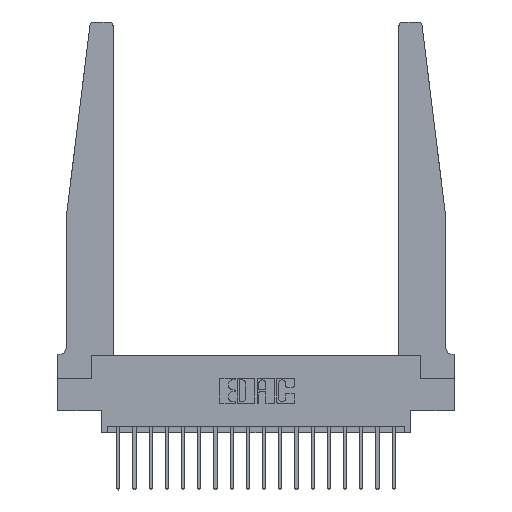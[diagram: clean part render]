
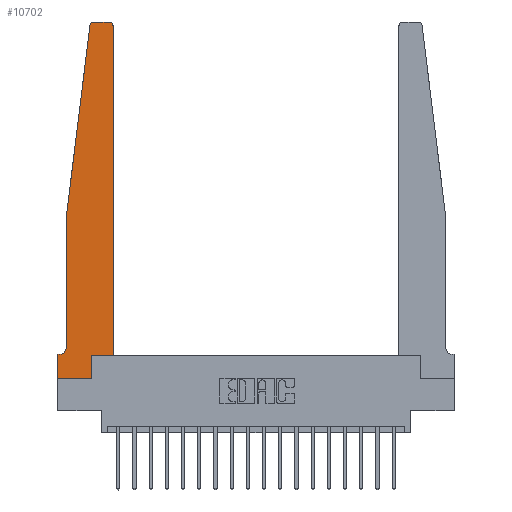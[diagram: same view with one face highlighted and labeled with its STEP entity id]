
A CAD part, top view. The second image highlights one B-rep face of the part: STEP entity #10702.
In plain terms, the highlighted planar face has unit normal (0, 0, 1).
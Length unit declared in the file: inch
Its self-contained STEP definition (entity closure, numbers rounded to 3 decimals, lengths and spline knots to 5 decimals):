
#874 = DIRECTION ( 'NONE',  ( -1., 0., 0. ) ) ;
#883 = VERTEX_POINT ( 'NONE', #2435 ) ;
#972 = CARTESIAN_POINT ( 'NONE',  ( 0., 0., 0.37 ) ) ;
#1206 = CARTESIAN_POINT ( 'NONE',  ( 0.065, 1.25, 0.37 ) ) ;
#1509 = CARTESIAN_POINT ( 'NONE',  ( 0.425, 0.18, 0.37 ) ) ;
#1638 = CARTESIAN_POINT ( 'NONE',  ( 0., 0.1875, 0.37 ) ) ;
#1744 = FACE_OUTER_BOUND ( 'NONE', #10239, .T. ) ;
#2054 = VECTOR ( 'NONE', #4395, 39.37008 ) ;
#2435 = CARTESIAN_POINT ( 'NONE',  ( 0.24675, 2.72367, 0.37 ) ) ;
#2833 = ORIENTED_EDGE ( 'NONE', *, *, #9319, .T. ) ;
#2853 = CARTESIAN_POINT ( 'NONE',  ( 0.425, 0.18, 0.37 ) ) ;
#2883 = LINE ( 'NONE', #19296, #9611 ) ;
#3149 = VECTOR ( 'NONE', #13732, 39.37008 ) ;
#3194 = DIRECTION ( 'NONE',  ( 1., 0., 0. ) ) ;
#3276 = CARTESIAN_POINT ( 'NONE',  ( 0.27653, 2.75, 0.37 ) ) ;
#3816 = ORIENTED_EDGE ( 'NONE', *, *, #16054, .T. ) ;
#4309 = VECTOR ( 'NONE', #18836, 39.37008 ) ;
#4395 = DIRECTION ( 'NONE',  ( 0., -1., 0. ) ) ;
#4402 = EDGE_CURVE ( 'NONE', #883, #15186, #13117, .T. ) ;
#4779 = AXIS2_PLACEMENT_3D ( 'NONE', #1638, #12386, #3194 ) ;
#5015 = ORIENTED_EDGE ( 'NONE', *, *, #6619, .T. ) ;
#5163 = CARTESIAN_POINT ( 'NONE',  ( 0.395, 2.72, 0.37 ) ) ;
#5362 = CARTESIAN_POINT ( 'NONE',  ( 0.27653, 2.72, 0.37 ) ) ;
#5660 = LINE ( 'NONE', #1206, #17437 ) ;
#5777 = CARTESIAN_POINT ( 'NONE',  ( 0.2605, 0.18, 0.37 ) ) ;
#5812 = CARTESIAN_POINT ( 'NONE',  ( 0.015, 0.2375, 0.37 ) ) ;
#5815 = EDGE_CURVE ( 'NONE', #15186, #13095, #5660, .T. ) ;
#5860 = CARTESIAN_POINT ( 'NONE',  ( 0., 0.1875, 0.37 ) ) ;
#6058 = CARTESIAN_POINT ( 'NONE',  ( 0.2605, 0., 0.37 ) ) ;
#6157 = VERTEX_POINT ( 'NONE', #19518 ) ;
#6160 = LINE ( 'NONE', #12027, #2054 ) ;
#6489 = CARTESIAN_POINT ( 'NONE',  ( 0.015, 0.1875, 0.37 ) ) ;
#6619 = EDGE_CURVE ( 'NONE', #15653, #883, #12093, .T. ) ;
#6700 = DIRECTION ( 'NONE',  ( 1., 0., 0. ) ) ;
#6887 = DIRECTION ( 'NONE',  ( 1., 0., 0. ) ) ;
#7202 = VECTOR ( 'NONE', #16511, 39.37008 ) ;
#7350 = DIRECTION ( 'NONE',  ( -1., 0., 0. ) ) ;
#7515 = DIRECTION ( 'NONE',  ( 1., 0., 0. ) ) ;
#7751 = LINE ( 'NONE', #12172, #3149 ) ;
#7836 = EDGE_CURVE ( 'NONE', #10323, #9070, #15899, .T. ) ;
#7864 = EDGE_CURVE ( 'NONE', #6157, #15653, #7751, .T. ) ;
#7906 = LINE ( 'NONE', #17312, #4309 ) ;
#8312 = EDGE_CURVE ( 'NONE', #13095, #19140, #11800, .T. ) ;
#8371 = EDGE_CURVE ( 'NONE', #8927, #10507, #6160, .T. ) ;
#8393 = ORIENTED_EDGE ( 'NONE', *, *, #16707, .T. ) ;
#8426 = VERTEX_POINT ( 'NONE', #6058 ) ;
#8843 = LINE ( 'NONE', #18296, #17024 ) ;
#8864 = ORIENTED_EDGE ( 'NONE', *, *, #15495, .T. ) ;
#8927 = VERTEX_POINT ( 'NONE', #5860 ) ;
#9070 = VERTEX_POINT ( 'NONE', #1509 ) ;
#9095 = DIRECTION ( 'NONE',  ( 1., 0., 0. ) ) ;
#9319 = EDGE_CURVE ( 'NONE', #16487, #6157, #14566, .T. ) ;
#9476 = CARTESIAN_POINT ( 'NONE',  ( 0.065, 0.2375, 0.37 ) ) ;
#9611 = VECTOR ( 'NONE', #874, 39.37008 ) ;
#10239 = EDGE_LOOP ( 'NONE', ( #13647, #5015, #16781, #12194, #19846, #8864, #12434, #8393, #3816, #19637, #15107, #2833 ) ) ;
#10323 = VERTEX_POINT ( 'NONE', #11480 ) ;
#10396 = DIRECTION ( 'NONE',  ( -0.122, -0.992, 0. ) ) ;
#10507 = VERTEX_POINT ( 'NONE', #972 ) ;
#10702 = ADVANCED_FACE ( 'NONE', ( #1744 ), #12323, .T. ) ;
#10782 = LINE ( 'NONE', #5777, #7202 ) ;
#11480 = CARTESIAN_POINT ( 'NONE',  ( 0.2605, 0.18, 0.37 ) ) ;
#11800 = CIRCLE ( 'NONE', #16057, 0.05 ) ;
#11821 = VECTOR ( 'NONE', #7515, 39.37008 ) ;
#12027 = CARTESIAN_POINT ( 'NONE',  ( 0., 0., 0.37 ) ) ;
#12093 = CIRCLE ( 'NONE', #17711, 0.03 ) ;
#12142 = VECTOR ( 'NONE', #10396, 39.37008 ) ;
#12172 = CARTESIAN_POINT ( 'NONE',  ( 0.25, 2.75, 0.37 ) ) ;
#12194 = ORIENTED_EDGE ( 'NONE', *, *, #5815, .T. ) ;
#12261 = CARTESIAN_POINT ( 'NONE',  ( 0.065, 1.25, 0.37 ) ) ;
#12323 = PLANE ( 'NONE',  #4779 ) ;
#12336 = DIRECTION ( 'NONE',  ( 0., -1., 0. ) ) ;
#12386 = DIRECTION ( 'NONE',  ( 0., 0., 1. ) ) ;
#12434 = ORIENTED_EDGE ( 'NONE', *, *, #8371, .T. ) ;
#13095 = VERTEX_POINT ( 'NONE', #9476 ) ;
#13117 = LINE ( 'NONE', #16513, #12142 ) ;
#13194 = CARTESIAN_POINT ( 'NONE',  ( 0.425, 2.72, 0.37 ) ) ;
#13647 = ORIENTED_EDGE ( 'NONE', *, *, #7864, .T. ) ;
#13732 = DIRECTION ( 'NONE',  ( -1., 0., 0. ) ) ;
#13768 = EDGE_CURVE ( 'NONE', #9070, #16487, #7906, .T. ) ;
#14566 = CIRCLE ( 'NONE', #15939, 0.03 ) ;
#15107 = ORIENTED_EDGE ( 'NONE', *, *, #13768, .T. ) ;
#15186 = VERTEX_POINT ( 'NONE', #12261 ) ;
#15495 = EDGE_CURVE ( 'NONE', #19140, #8927, #2883, .T. ) ;
#15653 = VERTEX_POINT ( 'NONE', #3276 ) ;
#15897 = DIRECTION ( 'NONE',  ( 0., 0., 1. ) ) ;
#15899 = LINE ( 'NONE', #2853, #11821 ) ;
#15939 = AXIS2_PLACEMENT_3D ( 'NONE', #5163, #15897, #6700 ) ;
#16054 = EDGE_CURVE ( 'NONE', #8426, #10323, #10782, .T. ) ;
#16057 = AXIS2_PLACEMENT_3D ( 'NONE', #5812, #16537, #7350 ) ;
#16094 = DIRECTION ( 'NONE',  ( 0., 0., 1. ) ) ;
#16487 = VERTEX_POINT ( 'NONE', #13194 ) ;
#16511 = DIRECTION ( 'NONE',  ( 0., 1., 0. ) ) ;
#16513 = CARTESIAN_POINT ( 'NONE',  ( 0.065, 1.25, 0.37 ) ) ;
#16537 = DIRECTION ( 'NONE',  ( 0., 0., -1. ) ) ;
#16707 = EDGE_CURVE ( 'NONE', #10507, #8426, #8843, .T. ) ;
#16781 = ORIENTED_EDGE ( 'NONE', *, *, #4402, .T. ) ;
#17024 = VECTOR ( 'NONE', #9095, 39.37008 ) ;
#17312 = CARTESIAN_POINT ( 'NONE',  ( 0.425, 0.18, 0.37 ) ) ;
#17437 = VECTOR ( 'NONE', #12336, 39.37008 ) ;
#17711 = AXIS2_PLACEMENT_3D ( 'NONE', #5362, #16094, #6887 ) ;
#18296 = CARTESIAN_POINT ( 'NONE',  ( 0., 0., 0.37 ) ) ;
#18836 = DIRECTION ( 'NONE',  ( 0., 1., 0. ) ) ;
#19140 = VERTEX_POINT ( 'NONE', #6489 ) ;
#19296 = CARTESIAN_POINT ( 'NONE',  ( 0.065, 0.1875, 0.37 ) ) ;
#19518 = CARTESIAN_POINT ( 'NONE',  ( 0.395, 2.75, 0.37 ) ) ;
#19637 = ORIENTED_EDGE ( 'NONE', *, *, #7836, .T. ) ;
#19846 = ORIENTED_EDGE ( 'NONE', *, *, #8312, .T. ) ;
